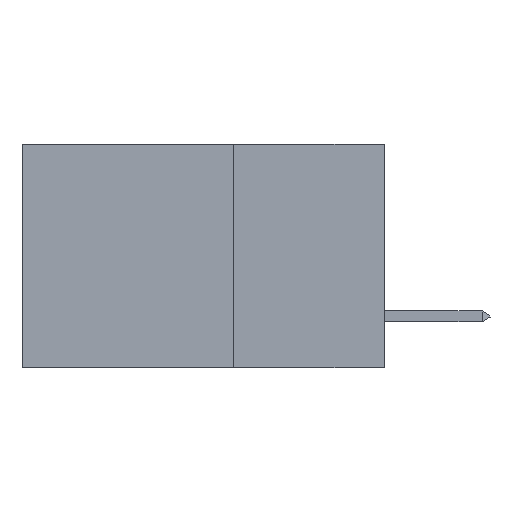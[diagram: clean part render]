
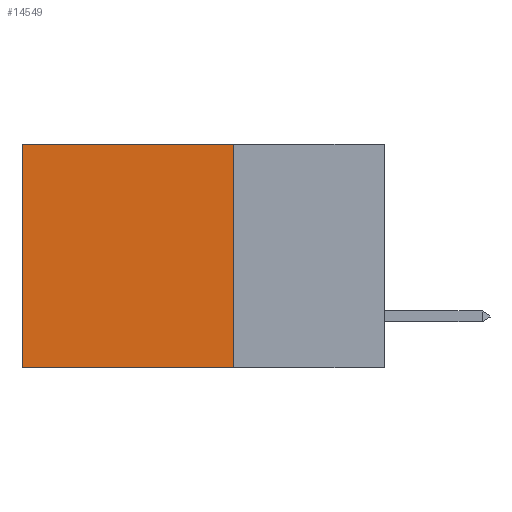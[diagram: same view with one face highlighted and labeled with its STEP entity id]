
A CAD part, left-side view. The second image highlights one B-rep face of the part: STEP entity #14549.
In plain terms, the highlighted planar face has unit normal (-1, 0, 0).
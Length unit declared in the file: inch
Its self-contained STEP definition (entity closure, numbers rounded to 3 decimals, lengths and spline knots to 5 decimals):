
#9 = VECTOR ( 'NONE', #16279, 39.37008 ) ;
#435 = LINE ( 'NONE', #8275, #9 ) ;
#515 = ORIENTED_EDGE ( 'NONE', *, *, #5654, .T. ) ;
#745 = ORIENTED_EDGE ( 'NONE', *, *, #3964, .F. ) ;
#1166 = CARTESIAN_POINT ( 'NONE',  ( 0.2875, 0.25, 0. ) ) ;
#1448 = DIRECTION ( 'NONE',  ( 0., 1., 0. ) ) ;
#1937 = CARTESIAN_POINT ( 'NONE',  ( 0.2875, 0.6, -0.37 ) ) ;
#2107 = CARTESIAN_POINT ( 'NONE',  ( 0.2875, 0.6, 0. ) ) ;
#3296 = DIRECTION ( 'NONE',  ( 0., 0., -1. ) ) ;
#3354 = PLANE ( 'NONE',  #10635 ) ;
#3611 = EDGE_CURVE ( 'NONE', #17340, #12631, #15720, .T. ) ;
#3964 = EDGE_CURVE ( 'NONE', #4565, #14268, #16348, .T. ) ;
#4565 = VERTEX_POINT ( 'NONE', #8964 ) ;
#4860 = LINE ( 'NONE', #9811, #9940 ) ;
#5654 = EDGE_CURVE ( 'NONE', #4565, #17340, #435, .T. ) ;
#7259 = DIRECTION ( 'NONE',  ( 0., 0., -1. ) ) ;
#8275 = CARTESIAN_POINT ( 'NONE',  ( 0.2875, 0.25, 0. ) ) ;
#8559 = FACE_OUTER_BOUND ( 'NONE', #12908, .T. ) ;
#8964 = CARTESIAN_POINT ( 'NONE',  ( 0.2875, 0.25, 0. ) ) ;
#9811 = CARTESIAN_POINT ( 'NONE',  ( 0.2875, 0.25, -0.37 ) ) ;
#9940 = VECTOR ( 'NONE', #1448, 39.37008 ) ;
#10635 = AXIS2_PLACEMENT_3D ( 'NONE', #14087, #16752, #3296 ) ;
#10862 = VECTOR ( 'NONE', #7259, 39.37008 ) ;
#11146 = EDGE_CURVE ( 'NONE', #14268, #12631, #4860, .T. ) ;
#12631 = VERTEX_POINT ( 'NONE', #1937 ) ;
#12692 = CARTESIAN_POINT ( 'NONE',  ( 0.2875, 0.6, 0. ) ) ;
#12908 = EDGE_LOOP ( 'NONE', ( #15815, #16376, #745, #515 ) ) ;
#12939 = VECTOR ( 'NONE', #15129, 39.37008 ) ;
#14087 = CARTESIAN_POINT ( 'NONE',  ( 0.2875, 0.25, 0. ) ) ;
#14268 = VERTEX_POINT ( 'NONE', #16638 ) ;
#14549 = ADVANCED_FACE ( 'NONE', ( #8559 ), #3354, .F. ) ;
#15129 = DIRECTION ( 'NONE',  ( 0., 0., -1. ) ) ;
#15720 = LINE ( 'NONE', #2107, #10862 ) ;
#15815 = ORIENTED_EDGE ( 'NONE', *, *, #3611, .T. ) ;
#16279 = DIRECTION ( 'NONE',  ( 0., 1., 0. ) ) ;
#16348 = LINE ( 'NONE', #1166, #12939 ) ;
#16376 = ORIENTED_EDGE ( 'NONE', *, *, #11146, .F. ) ;
#16638 = CARTESIAN_POINT ( 'NONE',  ( 0.2875, 0.25, -0.37 ) ) ;
#16752 = DIRECTION ( 'NONE',  ( 1., 0., 0. ) ) ;
#17340 = VERTEX_POINT ( 'NONE', #12692 ) ;
